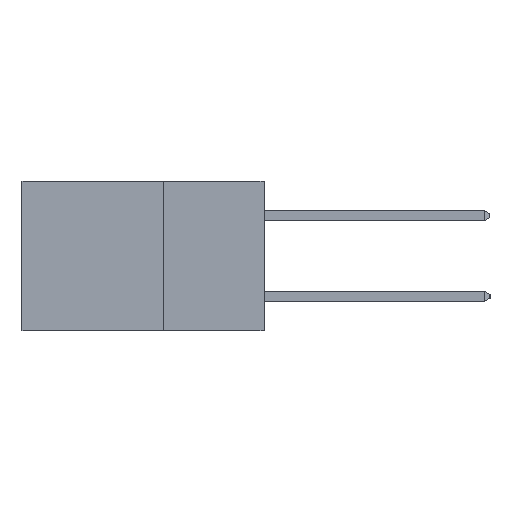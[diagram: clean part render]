
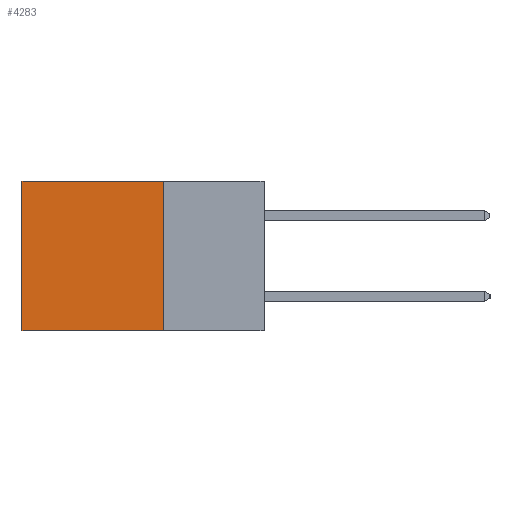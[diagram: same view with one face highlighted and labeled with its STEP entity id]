
A CAD part, left-side view. The second image highlights one B-rep face of the part: STEP entity #4283.
In plain terms, the highlighted planar face has unit normal (-1, 0, 0).
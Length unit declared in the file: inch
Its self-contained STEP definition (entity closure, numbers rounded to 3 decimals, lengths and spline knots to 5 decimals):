
#430 = VERTEX_POINT ( 'NONE', #2944 ) ;
#845 = DIRECTION ( 'NONE',  ( 0., 1., 0. ) ) ;
#1014 = CARTESIAN_POINT ( 'NONE',  ( 0.2615, 0.25, 0. ) ) ;
#1665 = ORIENTED_EDGE ( 'NONE', *, *, #7158, .T. ) ;
#2106 = DIRECTION ( 'NONE',  ( 0., 1., 0. ) ) ;
#2201 = DIRECTION ( 'NONE',  ( 0., 0., -1. ) ) ;
#2294 = DIRECTION ( 'NONE',  ( 1., 0., 0. ) ) ;
#2386 = CARTESIAN_POINT ( 'NONE',  ( 0.2615, 0.25, 0. ) ) ;
#2545 = LINE ( 'NONE', #3530, #16036 ) ;
#2579 = CARTESIAN_POINT ( 'NONE',  ( 0.2615, 0.25, -0.37 ) ) ;
#2623 = PLANE ( 'NONE',  #14668 ) ;
#2944 = CARTESIAN_POINT ( 'NONE',  ( 0.2615, 0.6, -0.37 ) ) ;
#2963 = ORIENTED_EDGE ( 'NONE', *, *, #3719, .F. ) ;
#3282 = VERTEX_POINT ( 'NONE', #2386 ) ;
#3287 = VECTOR ( 'NONE', #15885, 39.37008 ) ;
#3364 = DIRECTION ( 'NONE',  ( 0., 0., -1. ) ) ;
#3523 = VERTEX_POINT ( 'NONE', #9834 ) ;
#3530 = CARTESIAN_POINT ( 'NONE',  ( 0.2615, 0.6, -0.37 ) ) ;
#3719 = EDGE_CURVE ( 'NONE', #3282, #3523, #14198, .T. ) ;
#3914 = LINE ( 'NONE', #1014, #14007 ) ;
#4117 = CARTESIAN_POINT ( 'NONE',  ( 0.2615, 0.6, 0. ) ) ;
#4283 = ADVANCED_FACE ( 'NONE', ( #12167 ), #2623, .F. ) ;
#7158 = EDGE_CURVE ( 'NONE', #11761, #430, #2545, .T. ) ;
#7348 = EDGE_LOOP ( 'NONE', ( #1665, #13785, #2963, #13081 ) ) ;
#7437 = CARTESIAN_POINT ( 'NONE',  ( 0.2615, 0.25, -0.37 ) ) ;
#9524 = EDGE_CURVE ( 'NONE', #3282, #11761, #3914, .T. ) ;
#9834 = CARTESIAN_POINT ( 'NONE',  ( 0.2615, 0.25, -0.37 ) ) ;
#10904 = VECTOR ( 'NONE', #2106, 39.37008 ) ;
#11761 = VERTEX_POINT ( 'NONE', #4117 ) ;
#12167 = FACE_OUTER_BOUND ( 'NONE', #7348, .T. ) ;
#12906 = EDGE_CURVE ( 'NONE', #3523, #430, #13513, .T. ) ;
#13081 = ORIENTED_EDGE ( 'NONE', *, *, #9524, .T. ) ;
#13513 = LINE ( 'NONE', #7437, #10904 ) ;
#13785 = ORIENTED_EDGE ( 'NONE', *, *, #12906, .F. ) ;
#14007 = VECTOR ( 'NONE', #845, 39.37008 ) ;
#14198 = LINE ( 'NONE', #15920, #3287 ) ;
#14668 = AXIS2_PLACEMENT_3D ( 'NONE', #2579, #2294, #2201 ) ;
#15885 = DIRECTION ( 'NONE',  ( 0., 0., -1. ) ) ;
#15920 = CARTESIAN_POINT ( 'NONE',  ( 0.2615, 0.25, -0.37 ) ) ;
#16036 = VECTOR ( 'NONE', #3364, 39.37008 ) ;
